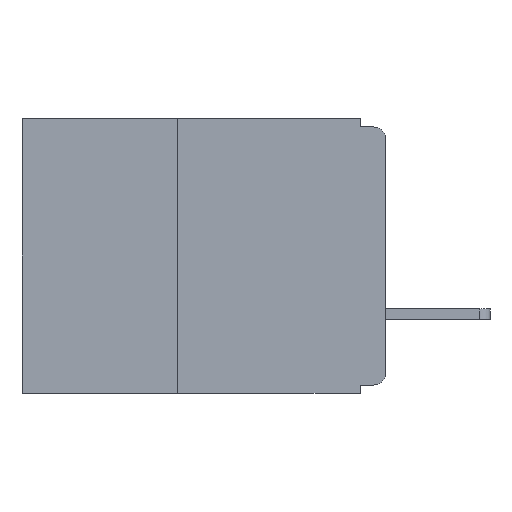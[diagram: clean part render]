
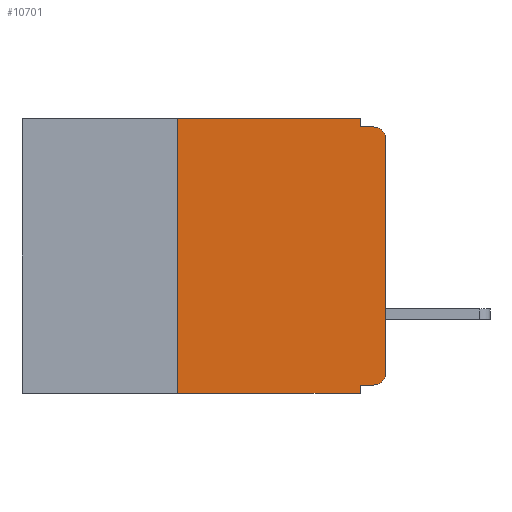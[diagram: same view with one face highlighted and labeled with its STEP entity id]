
A CAD part, left-side view. The second image highlights one B-rep face of the part: STEP entity #10701.
In plain terms, the highlighted planar face has unit normal (-1, 0, 0).
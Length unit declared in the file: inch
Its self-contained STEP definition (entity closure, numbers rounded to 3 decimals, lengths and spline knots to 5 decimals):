
#251 = VERTEX_POINT ( 'NONE', #5779 ) ;
#273 = EDGE_CURVE ( 'NONE', #3764, #18830, #12584, .T. ) ;
#279 = ORIENTED_EDGE ( 'NONE', *, *, #2994, .T. ) ;
#458 = FACE_OUTER_BOUND ( 'NONE', #10939, .T. ) ;
#970 = DIRECTION ( 'NONE',  ( -1., 0., 0. ) ) ;
#1111 = VERTEX_POINT ( 'NONE', #4318 ) ;
#1199 = ORIENTED_EDGE ( 'NONE', *, *, #273, .F. ) ;
#1214 = ORIENTED_EDGE ( 'NONE', *, *, #10795, .T. ) ;
#1262 = CARTESIAN_POINT ( 'NONE',  ( 0., 0., -0.01 ) ) ;
#1400 = VECTOR ( 'NONE', #17474, 39.37008 ) ;
#1536 = CARTESIAN_POINT ( 'NONE',  ( 0., 0.015, -0.01 ) ) ;
#2994 = EDGE_CURVE ( 'NONE', #1111, #8667, #12037, .T. ) ;
#3137 = EDGE_CURVE ( 'NONE', #13449, #21577, #14522, .T. ) ;
#3240 = EDGE_CURVE ( 'NONE', #3764, #4372, #16344, .T. ) ;
#3743 = ORIENTED_EDGE ( 'NONE', *, *, #17816, .F. ) ;
#3764 = VERTEX_POINT ( 'NONE', #4055 ) ;
#4055 = CARTESIAN_POINT ( 'NONE',  ( 0., 0.25, -0.33 ) ) ;
#4318 = CARTESIAN_POINT ( 'NONE',  ( 0., 0.015, -0.32 ) ) ;
#4372 = VERTEX_POINT ( 'NONE', #12173 ) ;
#5779 = CARTESIAN_POINT ( 'NONE',  ( 0., 0., -0.025 ) ) ;
#7000 = CARTESIAN_POINT ( 'NONE',  ( 0., 0., -0.32 ) ) ;
#7064 = VECTOR ( 'NONE', #7918, 39.37008 ) ;
#7447 = CARTESIAN_POINT ( 'NONE',  ( 0., 0.437, -0.33 ) ) ;
#7653 = CARTESIAN_POINT ( 'NONE',  ( 0., 0.437, 0. ) ) ;
#7918 = DIRECTION ( 'NONE',  ( 0., -1., 0. ) ) ;
#7952 = CARTESIAN_POINT ( 'NONE',  ( 0., 0., 0. ) ) ;
#8213 = AXIS2_PLACEMENT_3D ( 'NONE', #18784, #8451, #20520 ) ;
#8410 = EDGE_CURVE ( 'NONE', #18608, #4372, #10980, .T. ) ;
#8451 = DIRECTION ( 'NONE',  ( -1., 0., 0. ) ) ;
#8521 = LINE ( 'NONE', #15821, #17719 ) ;
#8667 = VERTEX_POINT ( 'NONE', #19874 ) ;
#8853 = CARTESIAN_POINT ( 'NONE',  ( 0., 0.031, -0.33 ) ) ;
#9404 = DIRECTION ( 'NONE',  ( 1., 0., 0. ) ) ;
#9702 = DIRECTION ( 'NONE',  ( 0., 0., 1. ) ) ;
#10002 = ORIENTED_EDGE ( 'NONE', *, *, #11819, .F. ) ;
#10162 = ORIENTED_EDGE ( 'NONE', *, *, #3240, .T. ) ;
#10565 = DIRECTION ( 'NONE',  ( 0., -1., 0. ) ) ;
#10701 = ADVANCED_FACE ( 'NONE', ( #458 ), #18019, .F. ) ;
#10795 = EDGE_CURVE ( 'NONE', #8667, #251, #12548, .T. ) ;
#10899 = VERTEX_POINT ( 'NONE', #18596 ) ;
#10939 = EDGE_LOOP ( 'NONE', ( #1214, #11003, #18184, #10002, #13524, #1199, #10162, #12698, #3743, #279 ) ) ;
#10980 = LINE ( 'NONE', #8853, #1400 ) ;
#11003 = ORIENTED_EDGE ( 'NONE', *, *, #13603, .T. ) ;
#11819 = EDGE_CURVE ( 'NONE', #10899, #13449, #20006, .T. ) ;
#11845 = DIRECTION ( 'NONE',  ( 0., 0., 1. ) ) ;
#11912 = CARTESIAN_POINT ( 'NONE',  ( 0., 0.25, -0.33 ) ) ;
#12013 = VECTOR ( 'NONE', #9702, 39.37008 ) ;
#12037 = CIRCLE ( 'NONE', #19651, 0.015 ) ;
#12173 = CARTESIAN_POINT ( 'NONE',  ( 0., 0.031, -0.33 ) ) ;
#12548 = LINE ( 'NONE', #7952, #12013 ) ;
#12584 = LINE ( 'NONE', #11912, #17144 ) ;
#12698 = ORIENTED_EDGE ( 'NONE', *, *, #8410, .F. ) ;
#13192 = CARTESIAN_POINT ( 'NONE',  ( 0., 0.031, -0.01 ) ) ;
#13449 = VERTEX_POINT ( 'NONE', #13192 ) ;
#13524 = ORIENTED_EDGE ( 'NONE', *, *, #19189, .F. ) ;
#13603 = EDGE_CURVE ( 'NONE', #251, #21577, #14098, .T. ) ;
#13946 = VECTOR ( 'NONE', #19827, 39.37008 ) ;
#14098 = CIRCLE ( 'NONE', #8213, 0.015 ) ;
#14211 = DIRECTION ( 'NONE',  ( 0., 0., -1. ) ) ;
#14522 = LINE ( 'NONE', #1262, #13946 ) ;
#15821 = CARTESIAN_POINT ( 'NONE',  ( 0., 0.437, 0. ) ) ;
#16344 = LINE ( 'NONE', #7447, #7064 ) ;
#17144 = VECTOR ( 'NONE', #11845, 39.37008 ) ;
#17474 = DIRECTION ( 'NONE',  ( 0., 0., -1. ) ) ;
#17719 = VECTOR ( 'NONE', #10565, 39.37008 ) ;
#17816 = EDGE_CURVE ( 'NONE', #1111, #18608, #19083, .T. ) ;
#18019 = PLANE ( 'NONE',  #18727 ) ;
#18184 = ORIENTED_EDGE ( 'NONE', *, *, #3137, .F. ) ;
#18537 = VECTOR ( 'NONE', #19198, 39.37008 ) ;
#18596 = CARTESIAN_POINT ( 'NONE',  ( 0., 0.031, 0. ) ) ;
#18608 = VERTEX_POINT ( 'NONE', #19252 ) ;
#18727 = AXIS2_PLACEMENT_3D ( 'NONE', #7653, #9404, #21420 ) ;
#18784 = CARTESIAN_POINT ( 'NONE',  ( 0., 0.015, -0.025 ) ) ;
#18830 = VERTEX_POINT ( 'NONE', #19925 ) ;
#19083 = LINE ( 'NONE', #7000, #18537 ) ;
#19189 = EDGE_CURVE ( 'NONE', #18830, #10899, #8521, .T. ) ;
#19198 = DIRECTION ( 'NONE',  ( 0., 1., 0. ) ) ;
#19252 = CARTESIAN_POINT ( 'NONE',  ( 0., 0.031, -0.32 ) ) ;
#19475 = VECTOR ( 'NONE', #14211, 39.37008 ) ;
#19651 = AXIS2_PLACEMENT_3D ( 'NONE', #21098, #970, #22317 ) ;
#19827 = DIRECTION ( 'NONE',  ( 0., -1., 0. ) ) ;
#19874 = CARTESIAN_POINT ( 'NONE',  ( 0., 0., -0.305 ) ) ;
#19925 = CARTESIAN_POINT ( 'NONE',  ( 0., 0.25, 0. ) ) ;
#20006 = LINE ( 'NONE', #22591, #19475 ) ;
#20520 = DIRECTION ( 'NONE',  ( 0., 0., -1. ) ) ;
#21098 = CARTESIAN_POINT ( 'NONE',  ( 0., 0.015, -0.305 ) ) ;
#21420 = DIRECTION ( 'NONE',  ( 0., 0., -1. ) ) ;
#21577 = VERTEX_POINT ( 'NONE', #1536 ) ;
#22317 = DIRECTION ( 'NONE',  ( 0., 0., -1. ) ) ;
#22591 = CARTESIAN_POINT ( 'NONE',  ( 0., 0.031, 0. ) ) ;
